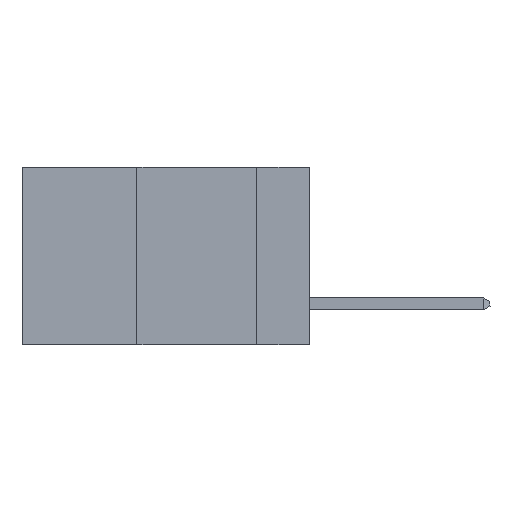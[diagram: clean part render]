
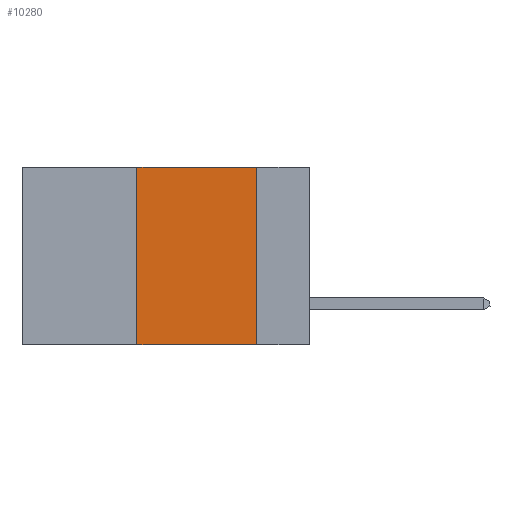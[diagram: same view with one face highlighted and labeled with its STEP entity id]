
A CAD part, left-side view. The second image highlights one B-rep face of the part: STEP entity #10280.
In plain terms, the highlighted planar face has unit normal (-1, 0, 0).
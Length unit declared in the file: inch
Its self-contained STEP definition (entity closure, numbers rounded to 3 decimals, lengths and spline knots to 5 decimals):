
#128 = DIRECTION ( 'NONE',  ( 0., 0., -1. ) ) ;
#678 = CARTESIAN_POINT ( 'NONE',  ( 0., 0.36, 0. ) ) ;
#1269 = ORIENTED_EDGE ( 'NONE', *, *, #2221, .T. ) ;
#1810 = ORIENTED_EDGE ( 'NONE', *, *, #6709, .F. ) ;
#2060 = VECTOR ( 'NONE', #7418, 39.37008 ) ;
#2218 = VERTEX_POINT ( 'NONE', #13940 ) ;
#2221 = EDGE_CURVE ( 'NONE', #2458, #13264, #2610, .T. ) ;
#2397 = CARTESIAN_POINT ( 'NONE',  ( 0., 0.6, -0.37 ) ) ;
#2458 = VERTEX_POINT ( 'NONE', #19223 ) ;
#2610 = LINE ( 'NONE', #2397, #2060 ) ;
#2944 = PLANE ( 'NONE',  #16196 ) ;
#4346 = VERTEX_POINT ( 'NONE', #20979 ) ;
#4443 = VECTOR ( 'NONE', #14023, 39.37008 ) ;
#4529 = EDGE_LOOP ( 'NONE', ( #11197, #10717, #1810, #1269 ) ) ;
#4652 = DIRECTION ( 'NONE',  ( 0., 0., -1. ) ) ;
#6613 = LINE ( 'NONE', #18085, #15799 ) ;
#6709 = EDGE_CURVE ( 'NONE', #2458, #4346, #8838, .T. ) ;
#7418 = DIRECTION ( 'NONE',  ( 0., -1., 0. ) ) ;
#7890 = CARTESIAN_POINT ( 'NONE',  ( 0., 0.6, 0. ) ) ;
#8838 = LINE ( 'NONE', #678, #4443 ) ;
#10186 = CARTESIAN_POINT ( 'NONE',  ( 0., 0.11, -0.37 ) ) ;
#10280 = ADVANCED_FACE ( 'NONE', ( #17482 ), #2944, .F. ) ;
#10717 = ORIENTED_EDGE ( 'NONE', *, *, #18961, .F. ) ;
#11197 = ORIENTED_EDGE ( 'NONE', *, *, #12658, .F. ) ;
#12658 = EDGE_CURVE ( 'NONE', #2218, #13264, #12889, .T. ) ;
#12889 = LINE ( 'NONE', #15072, #17135 ) ;
#13264 = VERTEX_POINT ( 'NONE', #10186 ) ;
#13940 = CARTESIAN_POINT ( 'NONE',  ( 0., 0.11, 0. ) ) ;
#14023 = DIRECTION ( 'NONE',  ( 0., 0., 1. ) ) ;
#14456 = DIRECTION ( 'NONE',  ( 1., 0., 0. ) ) ;
#15072 = CARTESIAN_POINT ( 'NONE',  ( 0., 0.11, 0. ) ) ;
#15799 = VECTOR ( 'NONE', #19679, 39.37008 ) ;
#16196 = AXIS2_PLACEMENT_3D ( 'NONE', #7890, #14456, #4652 ) ;
#17135 = VECTOR ( 'NONE', #128, 39.37008 ) ;
#17482 = FACE_OUTER_BOUND ( 'NONE', #4529, .T. ) ;
#18085 = CARTESIAN_POINT ( 'NONE',  ( 0., 0.6, 0. ) ) ;
#18961 = EDGE_CURVE ( 'NONE', #4346, #2218, #6613, .T. ) ;
#19223 = CARTESIAN_POINT ( 'NONE',  ( 0., 0.36, -0.37 ) ) ;
#19679 = DIRECTION ( 'NONE',  ( 0., -1., 0. ) ) ;
#20979 = CARTESIAN_POINT ( 'NONE',  ( 0., 0.36, 0. ) ) ;
